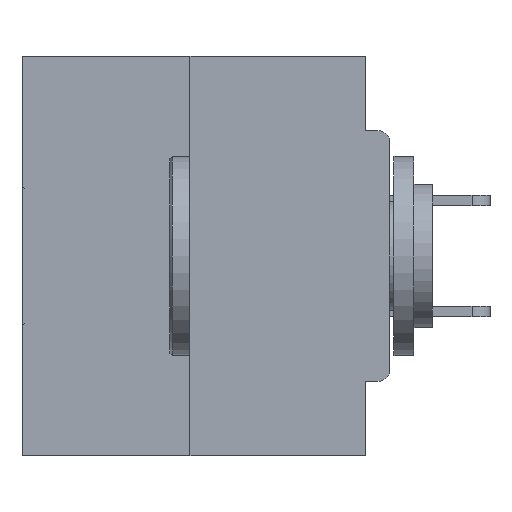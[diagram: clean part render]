
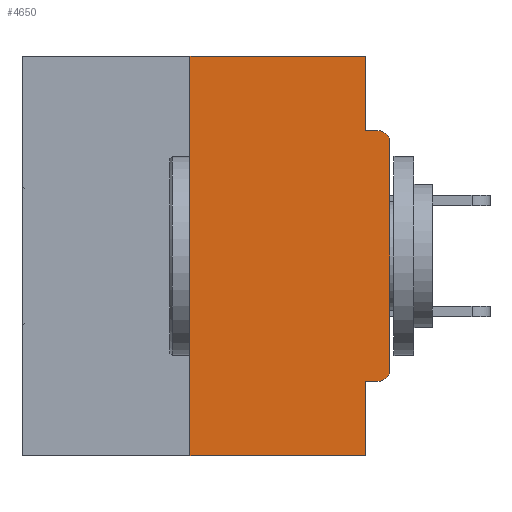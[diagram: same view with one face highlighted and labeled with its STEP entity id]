
A CAD part, left-side view. The second image highlights one B-rep face of the part: STEP entity #4650.
In plain terms, the highlighted planar face has unit normal (-1, 0, 0).
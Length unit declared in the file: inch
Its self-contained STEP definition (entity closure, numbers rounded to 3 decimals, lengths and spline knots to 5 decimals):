
#231 = ORIENTED_EDGE ( 'NONE', *, *, #6314, .F. ) ;
#1684 = LINE ( 'NONE', #17804, #4705 ) ;
#1916 = EDGE_CURVE ( 'NONE', #25032, #12980, #36320, .T. ) ;
#2358 = EDGE_CURVE ( 'NONE', #35516, #10890, #14639, .T. ) ;
#2605 = CARTESIAN_POINT ( 'NONE',  ( 0., 0., -0.4065 ) ) ;
#3226 = VERTEX_POINT ( 'NONE', #40060 ) ;
#3439 = LINE ( 'NONE', #22011, #25066 ) ;
#3950 = EDGE_CURVE ( 'NONE', #21506, #25032, #3439, .T. ) ;
#4650 = ADVANCED_FACE ( 'NONE', ( #16948 ), #13370, .F. ) ;
#4705 = VECTOR ( 'NONE', #4835, 39.37008 ) ;
#4835 = DIRECTION ( 'NONE',  ( 0., 0., 1. ) ) ;
#6314 = EDGE_CURVE ( 'NONE', #26517, #3226, #1684, .T. ) ;
#6354 = ORIENTED_EDGE ( 'NONE', *, *, #22395, .T. ) ;
#6476 = AXIS2_PLACEMENT_3D ( 'NONE', #26982, #16445, #22947 ) ;
#6789 = CARTESIAN_POINT ( 'NONE',  ( 0., 0.25, -0.5 ) ) ;
#8799 = CARTESIAN_POINT ( 'NONE',  ( 0., 0.015, -0.4065 ) ) ;
#9204 = DIRECTION ( 'NONE',  ( 0., 1., 0. ) ) ;
#9250 = DIRECTION ( 'NONE',  ( 0., 0., -1. ) ) ;
#9303 = CARTESIAN_POINT ( 'NONE',  ( 0., 0.031, 0. ) ) ;
#9825 = VECTOR ( 'NONE', #18548, 39.37008 ) ;
#10036 = CARTESIAN_POINT ( 'NONE',  ( 0., 0.031, -0.4065 ) ) ;
#10890 = VERTEX_POINT ( 'NONE', #31624 ) ;
#12616 = CARTESIAN_POINT ( 'NONE',  ( 0., 0., -0.3915 ) ) ;
#12980 = VERTEX_POINT ( 'NONE', #13032 ) ;
#13032 = CARTESIAN_POINT ( 'NONE',  ( 0., 0.015, -0.0935 ) ) ;
#13370 = PLANE ( 'NONE',  #6476 ) ;
#14393 = EDGE_LOOP ( 'NONE', ( #41468, #231, #18160, #14446, #40211, #18410, #41272, #6354, #14769, #37445 ) ) ;
#14446 = ORIENTED_EDGE ( 'NONE', *, *, #24933, .F. ) ;
#14639 = LINE ( 'NONE', #37005, #18159 ) ;
#14769 = ORIENTED_EDGE ( 'NONE', *, *, #1916, .F. ) ;
#14946 = DIRECTION ( 'NONE',  ( 0., 0., -1. ) ) ;
#16192 = VECTOR ( 'NONE', #27770, 39.37008 ) ;
#16445 = DIRECTION ( 'NONE',  ( 1., 0., 0. ) ) ;
#16601 = DIRECTION ( 'NONE',  ( -1., 0., 0. ) ) ;
#16948 = FACE_OUTER_BOUND ( 'NONE', #14393, .T. ) ;
#17593 = EDGE_CURVE ( 'NONE', #33394, #35516, #19936, .T. ) ;
#17804 = CARTESIAN_POINT ( 'NONE',  ( 0., 0.25, 0. ) ) ;
#17990 = AXIS2_PLACEMENT_3D ( 'NONE', #29537, #16601, #23092 ) ;
#18111 = CARTESIAN_POINT ( 'NONE',  ( 0., 0., -0.0935 ) ) ;
#18159 = VECTOR ( 'NONE', #30165, 39.37008 ) ;
#18160 = ORIENTED_EDGE ( 'NONE', *, *, #35885, .T. ) ;
#18410 = ORIENTED_EDGE ( 'NONE', *, *, #17593, .T. ) ;
#18548 = DIRECTION ( 'NONE',  ( 0., -1., 0. ) ) ;
#19097 = DIRECTION ( 'NONE',  ( 0., -1., 0. ) ) ;
#19322 = DIRECTION ( 'NONE',  ( 0., 0., -1. ) ) ;
#19936 = CIRCLE ( 'NONE', #31905, 0.015 ) ;
#21506 = VERTEX_POINT ( 'NONE', #9303 ) ;
#22011 = CARTESIAN_POINT ( 'NONE',  ( 0., 0.031, 0. ) ) ;
#22217 = LINE ( 'NONE', #25440, #30293 ) ;
#22395 = EDGE_CURVE ( 'NONE', #10890, #12980, #37644, .T. ) ;
#22551 = LINE ( 'NONE', #28205, #28034 ) ;
#22716 = EDGE_CURVE ( 'NONE', #3226, #21506, #22551, .T. ) ;
#22837 = VERTEX_POINT ( 'NONE', #10036 ) ;
#22947 = DIRECTION ( 'NONE',  ( 0., 0., -1. ) ) ;
#23092 = DIRECTION ( 'NONE',  ( 0., 0., -1. ) ) ;
#24049 = VECTOR ( 'NONE', #9204, 39.37008 ) ;
#24913 = CARTESIAN_POINT ( 'NONE',  ( 0., 0.031, -0.5 ) ) ;
#24933 = EDGE_CURVE ( 'NONE', #22837, #31062, #22217, .T. ) ;
#25032 = VERTEX_POINT ( 'NONE', #32463 ) ;
#25066 = VECTOR ( 'NONE', #19322, 39.37008 ) ;
#25440 = CARTESIAN_POINT ( 'NONE',  ( 0., 0.031, -0.5 ) ) ;
#26517 = VERTEX_POINT ( 'NONE', #6789 ) ;
#26982 = CARTESIAN_POINT ( 'NONE',  ( 0., 0.46, 0. ) ) ;
#27529 = CARTESIAN_POINT ( 'NONE',  ( 0., 0.46, -0.5 ) ) ;
#27770 = DIRECTION ( 'NONE',  ( 0., -1., 0. ) ) ;
#28034 = VECTOR ( 'NONE', #19097, 39.37008 ) ;
#28205 = CARTESIAN_POINT ( 'NONE',  ( 0., 0.46, 0. ) ) ;
#29537 = CARTESIAN_POINT ( 'NONE',  ( 0., 0.015, -0.1085 ) ) ;
#30165 = DIRECTION ( 'NONE',  ( 0., 0., 1. ) ) ;
#30293 = VECTOR ( 'NONE', #9250, 39.37008 ) ;
#31062 = VERTEX_POINT ( 'NONE', #24913 ) ;
#31093 = LINE ( 'NONE', #2605, #24049 ) ;
#31395 = DIRECTION ( 'NONE',  ( -1., 0., 0. ) ) ;
#31624 = CARTESIAN_POINT ( 'NONE',  ( 0., 0., -0.1085 ) ) ;
#31905 = AXIS2_PLACEMENT_3D ( 'NONE', #40898, #31395, #14946 ) ;
#32463 = CARTESIAN_POINT ( 'NONE',  ( 0., 0.031, -0.0935 ) ) ;
#33394 = VERTEX_POINT ( 'NONE', #8799 ) ;
#33471 = EDGE_CURVE ( 'NONE', #33394, #22837, #31093, .T. ) ;
#34956 = LINE ( 'NONE', #27529, #9825 ) ;
#35516 = VERTEX_POINT ( 'NONE', #12616 ) ;
#35885 = EDGE_CURVE ( 'NONE', #26517, #31062, #34956, .T. ) ;
#36320 = LINE ( 'NONE', #18111, #16192 ) ;
#37005 = CARTESIAN_POINT ( 'NONE',  ( 0., 0., 0. ) ) ;
#37445 = ORIENTED_EDGE ( 'NONE', *, *, #3950, .F. ) ;
#37644 = CIRCLE ( 'NONE', #17990, 0.015 ) ;
#40060 = CARTESIAN_POINT ( 'NONE',  ( 0., 0.25, 0. ) ) ;
#40211 = ORIENTED_EDGE ( 'NONE', *, *, #33471, .F. ) ;
#40898 = CARTESIAN_POINT ( 'NONE',  ( 0., 0.015, -0.3915 ) ) ;
#41272 = ORIENTED_EDGE ( 'NONE', *, *, #2358, .T. ) ;
#41468 = ORIENTED_EDGE ( 'NONE', *, *, #22716, .F. ) ;
